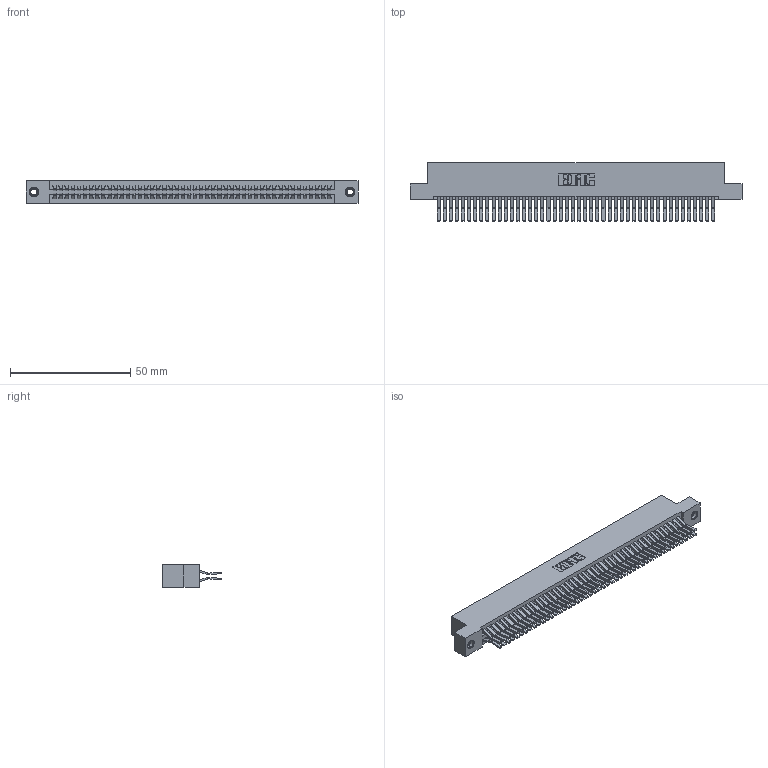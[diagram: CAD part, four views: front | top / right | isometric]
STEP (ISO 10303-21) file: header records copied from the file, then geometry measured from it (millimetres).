
FILE_DESCRIPTION (( 'STEP AP203' ), '1' );
FILE_NAME ('345-092-560-207.STEP', '2018-10-04T22:50:23', ( '' ), ( '' ), 'SwSTEP 2.0', 'SolidWorks 2016', '' );
FILE_SCHEMA (( 'CONFIG_CONTROL_DESIGN' ));
Length unit declared in the file: inch
Products named in the file (4): 345-250-001_345-250-005-103; 345-092-560-207; 345 Part_Flush Mounting Lugs - 0.156 Dia-TI; 345-292-001_560 Tail
Assembly tree (95 placements, depth 2):
  345-092-560-207
    345 Part_Flush Mounting Lugs - 0.156 Dia-TI
    345-292-001_560 Tail  x92
    345-250-001_345-250-005-103  x2
Bounding box: 138.05 x 24.45 x 9.4 mm (x, y, z)
Volume: 14036.9 mm3; surface area: 22405.1 mm2
Topology: 95 solids, 95 shells, 4970 faces, 14737 edges, 9694 vertices
Faces by surface type: plane 3148, cylinder 1806, cone 12, torus 4
Entity records: 36828 total; most frequent: CARTESIAN_POINT 6151, ORIENTED_EDGE 6078, DIRECTION 5449, EDGE_CURVE 3039, VECTOR 2699, LINE 2699, VERTEX_POINT 2020, AXIS2_PLACEMENT_3D 1375
